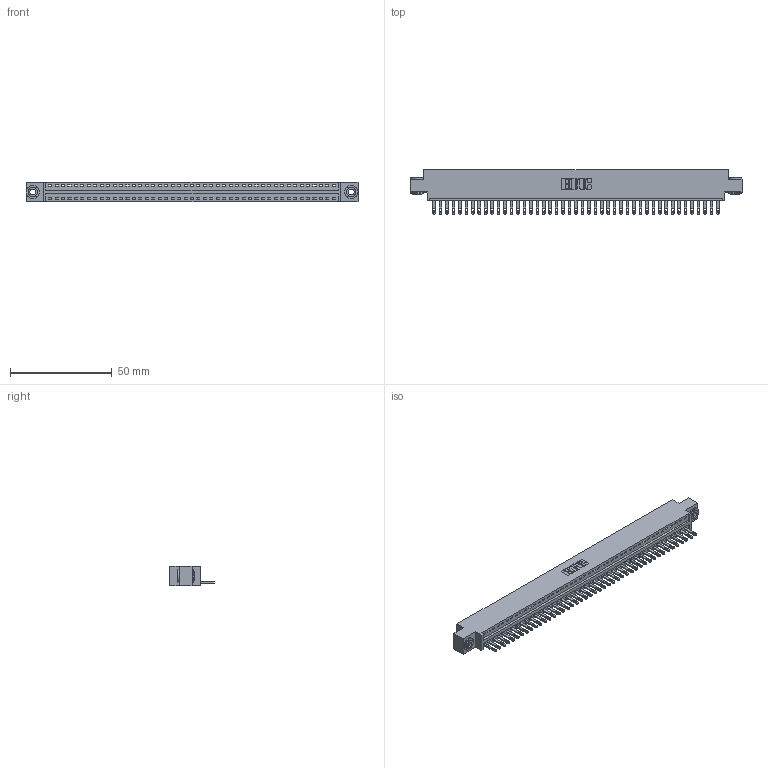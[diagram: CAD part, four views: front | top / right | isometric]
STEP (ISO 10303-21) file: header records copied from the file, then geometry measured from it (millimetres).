
FILE_DESCRIPTION (( 'STEP AP203' ), '1' );
FILE_NAME ('896-045-500-603.STEP', '2021-07-27T22:20:57', ( '' ), ( '' ), 'SwSTEP 2.0', 'SolidWorks 2020', '' );
FILE_SCHEMA (( 'CONFIG_CONTROL_DESIGN' ));
Length unit declared in the file: inch
Products named in the file (4): 846 Part_0.170 Offset - 0.156 Dia-TH; 345-292-001_345-293-100; 345-250-002_345-250-002-102; 896-045-500-603
Assembly tree (48 placements, depth 2):
  896-045-500-603
    846 Part_0.170 Offset - 0.156 Dia-TH
    345-292-001_345-293-100  x45
    345-250-002_345-250-002-102  x2
Bounding box: 163.45 x 21.84 x 9.4 mm (x, y, z)
Volume: 15559 mm3; surface area: 19963.5 mm2
Topology: 48 solids, 48 shells, 2594 faces, 7977 edges, 5314 vertices
Faces by surface type: plane 1620, cylinder 966, cone 8
Entity records: 28236 total; most frequent: CARTESIAN_POINT 4818, ORIENTED_EDGE 4790, DIRECTION 4279, EDGE_CURVE 2395, LINE 2055, VECTOR 2055, VERTEX_POINT 1594, AXIS2_PLACEMENT_3D 1112
